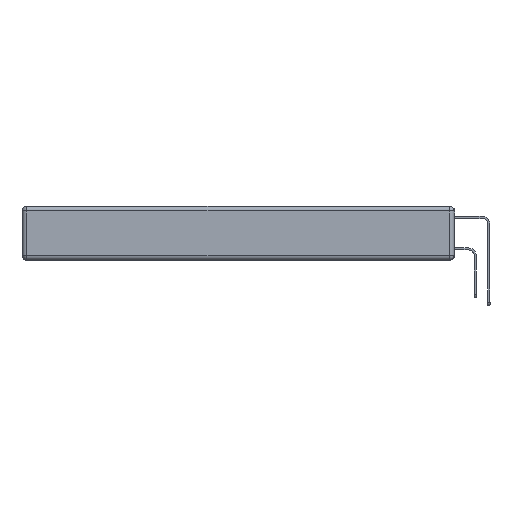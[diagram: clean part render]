
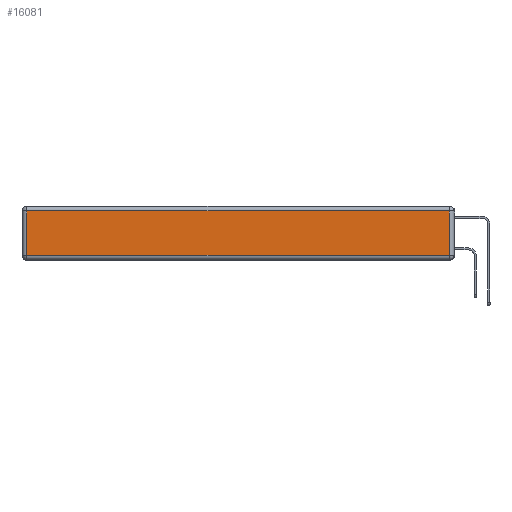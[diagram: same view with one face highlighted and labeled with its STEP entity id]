
A CAD part, left-side view. The second image highlights one B-rep face of the part: STEP entity #16081.
In plain terms, the highlighted planar face has unit normal (-1, 0, 0).
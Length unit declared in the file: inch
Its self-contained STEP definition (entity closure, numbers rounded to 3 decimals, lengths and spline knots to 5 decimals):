
#713 = DIRECTION ( 'NONE',  ( 0., 0., 1. ) ) ;
#816 = FACE_OUTER_BOUND ( 'NONE', #1980, .T. ) ;
#1418 = EDGE_CURVE ( 'NONE', #18178, #16154, #14183, .T. ) ;
#1980 = EDGE_LOOP ( 'NONE', ( #3364, #3865, #8594, #10797 ) ) ;
#2284 = DIRECTION ( 'NONE',  ( -1., 0., 0. ) ) ;
#3364 = ORIENTED_EDGE ( 'NONE', *, *, #6256, .T. ) ;
#3704 = LINE ( 'NONE', #19800, #10103 ) ;
#3865 = ORIENTED_EDGE ( 'NONE', *, *, #1418, .T. ) ;
#6030 = EDGE_CURVE ( 'NONE', #19955, #12882, #15668, .T. ) ;
#6256 = EDGE_CURVE ( 'NONE', #12882, #18178, #3704, .T. ) ;
#7666 = CARTESIAN_POINT ( 'NONE',  ( 0., 0.03, -0.03 ) ) ;
#8314 = CARTESIAN_POINT ( 'NONE',  ( 0., 2.75, -0.03 ) ) ;
#8594 = ORIENTED_EDGE ( 'NONE', *, *, #20131, .T. ) ;
#8596 = VECTOR ( 'NONE', #18941, 39.37008 ) ;
#9613 = VECTOR ( 'NONE', #12960, 39.37008 ) ;
#10103 = VECTOR ( 'NONE', #17038, 39.37008 ) ;
#10563 = CARTESIAN_POINT ( 'NONE',  ( 0., 2.72, -0.03 ) ) ;
#10797 = ORIENTED_EDGE ( 'NONE', *, *, #6030, .T. ) ;
#10916 = CARTESIAN_POINT ( 'NONE',  ( 0., 0.03, -0.343 ) ) ;
#12882 = VERTEX_POINT ( 'NONE', #17189 ) ;
#12960 = DIRECTION ( 'NONE',  ( 0., 1., 0. ) ) ;
#14183 = LINE ( 'NONE', #10916, #8596 ) ;
#15613 = AXIS2_PLACEMENT_3D ( 'NONE', #20351, #2284, #713 ) ;
#15668 = LINE ( 'NONE', #15877, #15902 ) ;
#15877 = CARTESIAN_POINT ( 'NONE',  ( 0., 2.72, -0.343 ) ) ;
#15902 = VECTOR ( 'NONE', #17474, 39.37008 ) ;
#16081 = ADVANCED_FACE ( 'NONE', ( #816 ), #16763, .T. ) ;
#16154 = VERTEX_POINT ( 'NONE', #7666 ) ;
#16763 = PLANE ( 'NONE',  #15613 ) ;
#17038 = DIRECTION ( 'NONE',  ( 0., -1., 0. ) ) ;
#17189 = CARTESIAN_POINT ( 'NONE',  ( 0., 2.72, -0.313 ) ) ;
#17474 = DIRECTION ( 'NONE',  ( 0., 0., -1. ) ) ;
#18178 = VERTEX_POINT ( 'NONE', #20000 ) ;
#18242 = LINE ( 'NONE', #8314, #9613 ) ;
#18941 = DIRECTION ( 'NONE',  ( 0., 0., 1. ) ) ;
#19800 = CARTESIAN_POINT ( 'NONE',  ( 0., 0., -0.313 ) ) ;
#19955 = VERTEX_POINT ( 'NONE', #10563 ) ;
#20000 = CARTESIAN_POINT ( 'NONE',  ( 0., 0.03, -0.313 ) ) ;
#20131 = EDGE_CURVE ( 'NONE', #16154, #19955, #18242, .T. ) ;
#20351 = CARTESIAN_POINT ( 'NONE',  ( 0., 0., -0.343 ) ) ;
